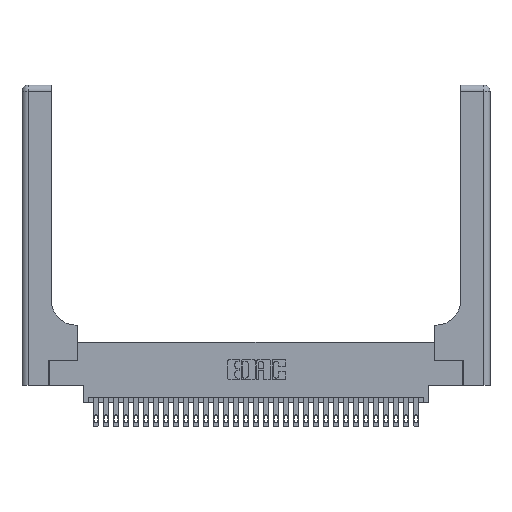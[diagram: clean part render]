
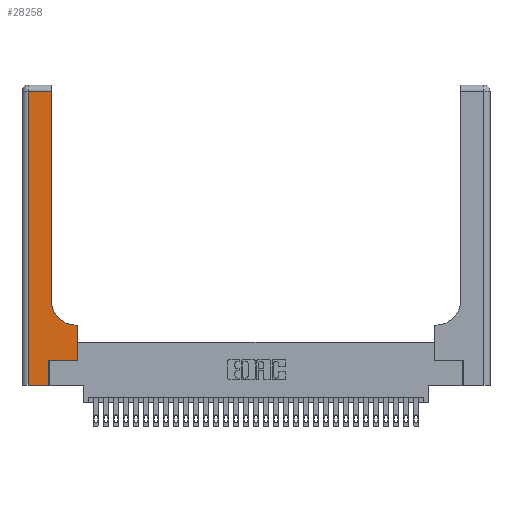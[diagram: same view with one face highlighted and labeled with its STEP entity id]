
A CAD part, top view. The second image highlights one B-rep face of the part: STEP entity #28258.
In plain terms, the highlighted planar face has unit normal (0, 0, 1).
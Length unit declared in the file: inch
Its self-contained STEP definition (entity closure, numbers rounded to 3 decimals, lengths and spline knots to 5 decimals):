
#316 = CARTESIAN_POINT ( 'NONE',  ( 0.269, 0.25, 0.37 ) ) ;
#454 = DIRECTION ( 'NONE',  ( 0., 0., -1. ) ) ;
#665 = DIRECTION ( 'NONE',  ( -1., 0., 0. ) ) ;
#2812 = CIRCLE ( 'NONE', #24000, 0.25 ) ;
#2871 = CARTESIAN_POINT ( 'NONE',  ( 0., 2.94, 0.37 ) ) ;
#3418 = CARTESIAN_POINT ( 'NONE',  ( 0.2915, 0.6, 0.37 ) ) ;
#3636 = VERTEX_POINT ( 'NONE', #9119 ) ;
#3991 = CARTESIAN_POINT ( 'NONE',  ( 0.269, 0., 0.37 ) ) ;
#4174 = CARTESIAN_POINT ( 'NONE',  ( 0.269, 0., 0.37 ) ) ;
#4533 = VECTOR ( 'NONE', #21119, 39.37008 ) ;
#5301 = CARTESIAN_POINT ( 'NONE',  ( 0., 3., 0.37 ) ) ;
#5690 = LINE ( 'NONE', #2871, #22909 ) ;
#5785 = DIRECTION ( 'NONE',  ( 0., -1., 0. ) ) ;
#5922 = VECTOR ( 'NONE', #26903, 39.37008 ) ;
#7174 = CARTESIAN_POINT ( 'NONE',  ( 0.06, 0., 0.37 ) ) ;
#8149 = DIRECTION ( 'NONE',  ( 0., 1., 0. ) ) ;
#8506 = CARTESIAN_POINT ( 'NONE',  ( 0.5415, 0.85, 0.37 ) ) ;
#8728 = ORIENTED_EDGE ( 'NONE', *, *, #19796, .T. ) ;
#8933 = VERTEX_POINT ( 'NONE', #18576 ) ;
#8945 = ORIENTED_EDGE ( 'NONE', *, *, #13109, .T. ) ;
#9119 = CARTESIAN_POINT ( 'NONE',  ( 0.5585, 0.6, 0.37 ) ) ;
#10678 = CARTESIAN_POINT ( 'NONE',  ( 0.2915, 0.85, 0.37 ) ) ;
#10924 = EDGE_CURVE ( 'NONE', #27919, #3636, #28854, .T. ) ;
#11004 = DIRECTION ( 'NONE',  ( 1., 0., 0. ) ) ;
#12218 = EDGE_CURVE ( 'NONE', #23089, #25146, #18735, .T. ) ;
#12584 = ORIENTED_EDGE ( 'NONE', *, *, #20677, .T. ) ;
#13109 = EDGE_CURVE ( 'NONE', #3636, #17359, #20956, .T. ) ;
#13434 = EDGE_CURVE ( 'NONE', #8933, #27919, #26537, .T. ) ;
#14011 = CARTESIAN_POINT ( 'NONE',  ( 0.5585, 0.25, 0.37 ) ) ;
#14016 = CARTESIAN_POINT ( 'NONE',  ( 0.2915, 2.94, 0.37 ) ) ;
#14102 = VECTOR ( 'NONE', #15456, 39.37008 ) ;
#14359 = VECTOR ( 'NONE', #22975, 39.37008 ) ;
#15441 = CARTESIAN_POINT ( 'NONE',  ( 0.06, 2.94, 0.37 ) ) ;
#15448 = EDGE_CURVE ( 'NONE', #25146, #18185, #26561, .T. ) ;
#15456 = DIRECTION ( 'NONE',  ( 1., 0., 0. ) ) ;
#16420 = ORIENTED_EDGE ( 'NONE', *, *, #13434, .T. ) ;
#17061 = AXIS2_PLACEMENT_3D ( 'NONE', #5301, #454, #17820 ) ;
#17359 = VERTEX_POINT ( 'NONE', #30756 ) ;
#17820 = DIRECTION ( 'NONE',  ( -1., 0., 0. ) ) ;
#17935 = VECTOR ( 'NONE', #5785, 39.37008 ) ;
#18077 = CARTESIAN_POINT ( 'NONE',  ( 0.06, 3., 0.37 ) ) ;
#18185 = VERTEX_POINT ( 'NONE', #3991 ) ;
#18576 = CARTESIAN_POINT ( 'NONE',  ( 0.269, 0.25, 0.37 ) ) ;
#18735 = LINE ( 'NONE', #18077, #17935 ) ;
#18901 = FACE_OUTER_BOUND ( 'NONE', #19722, .T. ) ;
#19032 = ORIENTED_EDGE ( 'NONE', *, *, #12218, .T. ) ;
#19400 = CARTESIAN_POINT ( 'NONE',  ( 0.2915, 3., 0.37 ) ) ;
#19722 = EDGE_LOOP ( 'NONE', ( #8728, #31771, #19032, #29422, #28858, #16420, #19781, #8945, #12584 ) ) ;
#19781 = ORIENTED_EDGE ( 'NONE', *, *, #10924, .T. ) ;
#19796 = EDGE_CURVE ( 'NONE', #27239, #31127, #20807, .T. ) ;
#20677 = EDGE_CURVE ( 'NONE', #17359, #27239, #2812, .T. ) ;
#20807 = LINE ( 'NONE', #19400, #5922 ) ;
#20811 = CARTESIAN_POINT ( 'NONE',  ( 0.5585, 0.25, 0.37 ) ) ;
#20956 = LINE ( 'NONE', #3418, #4533 ) ;
#21119 = DIRECTION ( 'NONE',  ( -1., 0., 0. ) ) ;
#22909 = VECTOR ( 'NONE', #665, 39.37008 ) ;
#22975 = DIRECTION ( 'NONE',  ( 1., 0., 0. ) ) ;
#23089 = VERTEX_POINT ( 'NONE', #15441 ) ;
#23233 = DIRECTION ( 'NONE',  ( 0., 0., -1. ) ) ;
#24000 = AXIS2_PLACEMENT_3D ( 'NONE', #8506, #23233, #11004 ) ;
#24595 = VECTOR ( 'NONE', #8149, 39.37008 ) ;
#25050 = VECTOR ( 'NONE', #26449, 39.37008 ) ;
#25146 = VERTEX_POINT ( 'NONE', #7174 ) ;
#25281 = EDGE_CURVE ( 'NONE', #31127, #23089, #5690, .T. ) ;
#26449 = DIRECTION ( 'NONE',  ( 0., 1., 0. ) ) ;
#26537 = LINE ( 'NONE', #316, #14359 ) ;
#26561 = LINE ( 'NONE', #30106, #14102 ) ;
#26903 = DIRECTION ( 'NONE',  ( 0., 1., 0. ) ) ;
#27003 = LINE ( 'NONE', #4174, #25050 ) ;
#27239 = VERTEX_POINT ( 'NONE', #10678 ) ;
#27919 = VERTEX_POINT ( 'NONE', #14011 ) ;
#28258 = ADVANCED_FACE ( 'NONE', ( #18901 ), #30383, .F. ) ;
#28854 = LINE ( 'NONE', #20811, #24595 ) ;
#28858 = ORIENTED_EDGE ( 'NONE', *, *, #28985, .T. ) ;
#28985 = EDGE_CURVE ( 'NONE', #18185, #8933, #27003, .T. ) ;
#29422 = ORIENTED_EDGE ( 'NONE', *, *, #15448, .T. ) ;
#30106 = CARTESIAN_POINT ( 'NONE',  ( 0., 0., 0.37 ) ) ;
#30383 = PLANE ( 'NONE',  #17061 ) ;
#30756 = CARTESIAN_POINT ( 'NONE',  ( 0.5415, 0.6, 0.37 ) ) ;
#31127 = VERTEX_POINT ( 'NONE', #14016 ) ;
#31771 = ORIENTED_EDGE ( 'NONE', *, *, #25281, .T. ) ;
